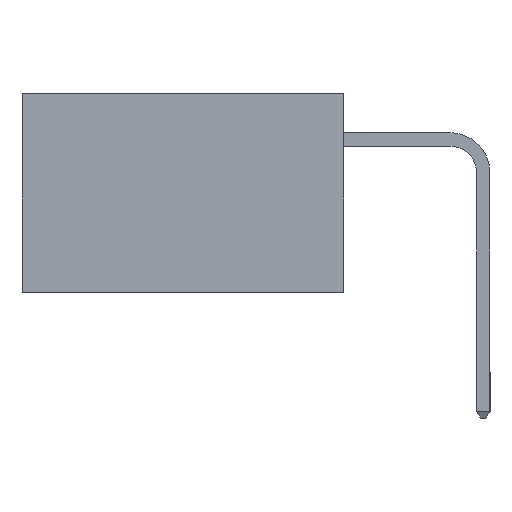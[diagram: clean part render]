
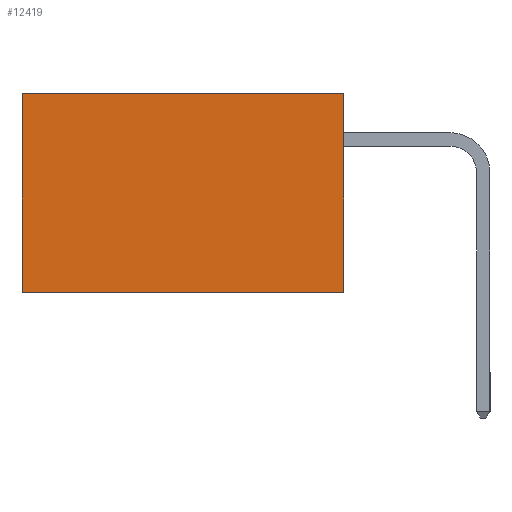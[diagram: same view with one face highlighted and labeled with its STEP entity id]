
A CAD part, left-side view. The second image highlights one B-rep face of the part: STEP entity #12419.
In plain terms, the highlighted planar face has unit normal (-1, 0, 0).
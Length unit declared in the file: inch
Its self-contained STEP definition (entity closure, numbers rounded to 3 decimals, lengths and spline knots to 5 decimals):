
#332 = CARTESIAN_POINT ( 'NONE',  ( 0.298, 0., 0. ) ) ;
#1156 = CARTESIAN_POINT ( 'NONE',  ( 0.298, 0., 0. ) ) ;
#1771 = VERTEX_POINT ( 'NONE', #11288 ) ;
#2099 = CARTESIAN_POINT ( 'NONE',  ( 0.298, 0.6, 0. ) ) ;
#2860 = EDGE_CURVE ( 'NONE', #12024, #9772, #10980, .T. ) ;
#3337 = DIRECTION ( 'NONE',  ( 0., 0., -1. ) ) ;
#3436 = CARTESIAN_POINT ( 'NONE',  ( 0.298, 0., 0. ) ) ;
#3813 = EDGE_LOOP ( 'NONE', ( #3858, #8610, #6757, #8743 ) ) ;
#3858 = ORIENTED_EDGE ( 'NONE', *, *, #8643, .T. ) ;
#5136 = LINE ( 'NONE', #3436, #9846 ) ;
#5765 = EDGE_CURVE ( 'NONE', #12024, #1771, #5136, .T. ) ;
#5948 = VECTOR ( 'NONE', #13290, 39.37008 ) ;
#6531 = CARTESIAN_POINT ( 'NONE',  ( 0.298, 0., 0. ) ) ;
#6757 = ORIENTED_EDGE ( 'NONE', *, *, #5765, .F. ) ;
#6797 = VERTEX_POINT ( 'NONE', #7733 ) ;
#6955 = DIRECTION ( 'NONE',  ( 0., 0., -1. ) ) ;
#6984 = FACE_OUTER_BOUND ( 'NONE', #3813, .T. ) ;
#6997 = PLANE ( 'NONE',  #10776 ) ;
#7004 = CARTESIAN_POINT ( 'NONE',  ( 0.298, 0., -0.37 ) ) ;
#7733 = CARTESIAN_POINT ( 'NONE',  ( 0.298, 0.6, -0.37 ) ) ;
#8331 = EDGE_CURVE ( 'NONE', #1771, #6797, #12187, .T. ) ;
#8610 = ORIENTED_EDGE ( 'NONE', *, *, #8331, .F. ) ;
#8643 = EDGE_CURVE ( 'NONE', #9772, #6797, #9693, .T. ) ;
#8743 = ORIENTED_EDGE ( 'NONE', *, *, #2860, .T. ) ;
#9276 = VECTOR ( 'NONE', #10252, 39.37008 ) ;
#9693 = LINE ( 'NONE', #14383, #14233 ) ;
#9772 = VERTEX_POINT ( 'NONE', #2099 ) ;
#9846 = VECTOR ( 'NONE', #3337, 39.37008 ) ;
#9937 = DIRECTION ( 'NONE',  ( 0., 0., -1. ) ) ;
#10252 = DIRECTION ( 'NONE',  ( 0., 1., 0. ) ) ;
#10776 = AXIS2_PLACEMENT_3D ( 'NONE', #332, #13614, #6955 ) ;
#10980 = LINE ( 'NONE', #6531, #5948 ) ;
#11288 = CARTESIAN_POINT ( 'NONE',  ( 0.298, 0., -0.37 ) ) ;
#12024 = VERTEX_POINT ( 'NONE', #1156 ) ;
#12187 = LINE ( 'NONE', #7004, #9276 ) ;
#12419 = ADVANCED_FACE ( 'NONE', ( #6984 ), #6997, .F. ) ;
#13290 = DIRECTION ( 'NONE',  ( 0., 1., 0. ) ) ;
#13614 = DIRECTION ( 'NONE',  ( 1., 0., 0. ) ) ;
#14233 = VECTOR ( 'NONE', #9937, 39.37008 ) ;
#14383 = CARTESIAN_POINT ( 'NONE',  ( 0.298, 0.6, 0. ) ) ;
